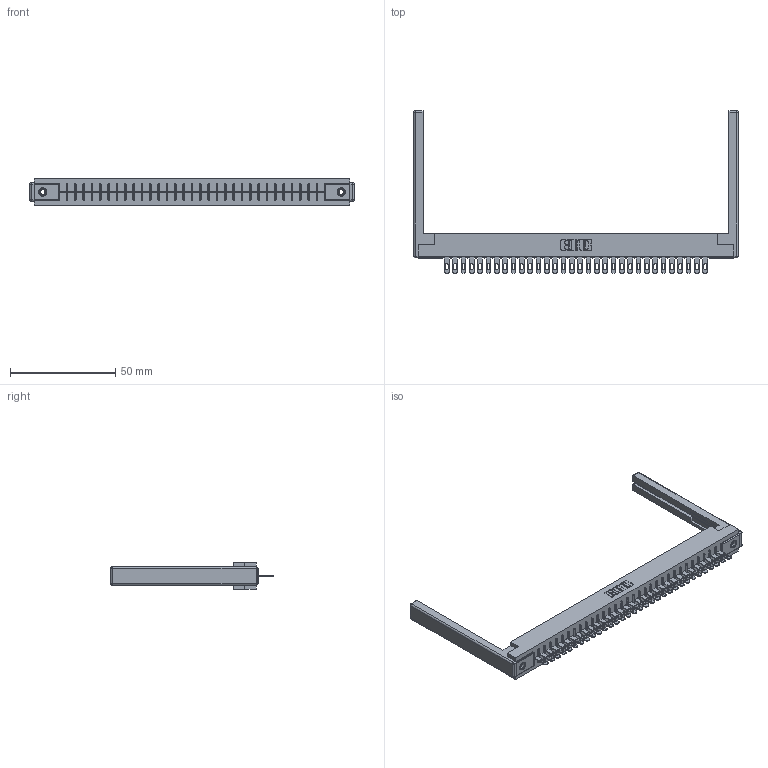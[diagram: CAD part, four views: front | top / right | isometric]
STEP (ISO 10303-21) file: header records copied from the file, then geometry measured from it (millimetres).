
FILE_DESCRIPTION (( 'STEP AP203' ), '1' );
FILE_NAME ('356-032-500-168.STEP', '2018-08-01T21:13:47', ( '' ), ( '' ), 'SwSTEP 2.0', 'SolidWorks 2016', '' );
FILE_SCHEMA (( 'CONFIG_CONTROL_DESIGN' ));
Length unit declared in the file: inch
Products named in the file (5): 306 Part_.156 Dia; 306-290-001_100; 345-250-001_345-250-001-102; 307-220-068; 356-032-500-168
Assembly tree (37 placements, depth 2):
  356-032-500-168
    306 Part_.156 Dia
    306-290-001_100  x32
    345-250-001_345-250-001-102  x2
    307-220-068  x2
Bounding box: 154.23 x 77.17 x 12.7 mm (x, y, z)
Volume: 21427.1 mm3; surface area: 22034.7 mm2
Topology: 37 solids, 37 shells, 2702 faces, 7586 edges, 4864 vertices
Faces by surface type: plane 1756, cylinder 794, sphere 136, cone 12, torus 4
Entity records: 34060 total; most frequent: CARTESIAN_POINT 5684, ORIENTED_EDGE 5626, DIRECTION 5619, EDGE_CURVE 2813, LINE 2189, VECTOR 2189, VERTEX_POINT 1780, AXIS2_PLACEMENT_3D 1715
